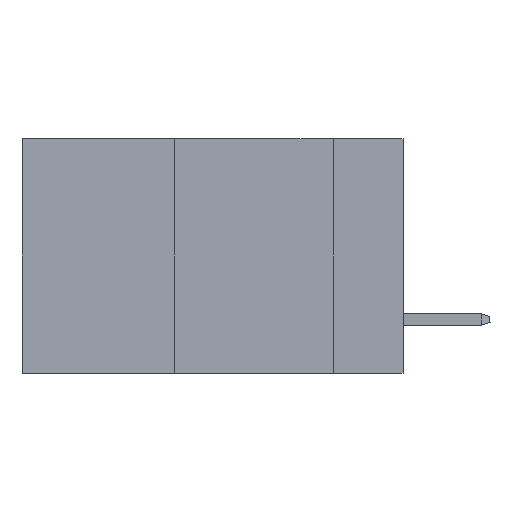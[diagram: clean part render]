
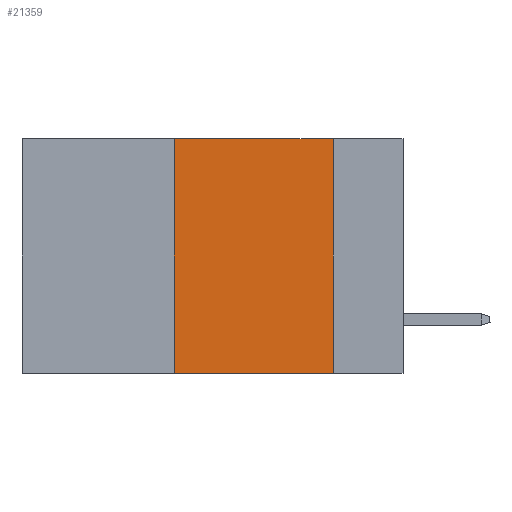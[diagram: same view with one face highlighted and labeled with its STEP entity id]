
A CAD part, left-side view. The second image highlights one B-rep face of the part: STEP entity #21359.
In plain terms, the highlighted planar face has unit normal (-1, 0, 0).
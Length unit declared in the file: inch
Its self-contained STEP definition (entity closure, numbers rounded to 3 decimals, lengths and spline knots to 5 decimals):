
#491 = CARTESIAN_POINT ( 'NONE',  ( 0., 0.36, 0. ) ) ;
#593 = CARTESIAN_POINT ( 'NONE',  ( 0., 0.6, -0.37 ) ) ;
#885 = ORIENTED_EDGE ( 'NONE', *, *, #23435, .F. ) ;
#1419 = CARTESIAN_POINT ( 'NONE',  ( 0., 0.36, 0. ) ) ;
#1528 = LINE ( 'NONE', #17895, #15842 ) ;
#1784 = VERTEX_POINT ( 'NONE', #1419 ) ;
#2158 = EDGE_CURVE ( 'NONE', #2268, #11792, #1528, .T. ) ;
#2268 = VERTEX_POINT ( 'NONE', #6514 ) ;
#4286 = DIRECTION ( 'NONE',  ( 1., 0., 0. ) ) ;
#4711 = LINE ( 'NONE', #491, #28111 ) ;
#5995 = LINE ( 'NONE', #21917, #21559 ) ;
#6258 = FACE_OUTER_BOUND ( 'NONE', #28922, .T. ) ;
#6408 = PLANE ( 'NONE',  #7653 ) ;
#6514 = CARTESIAN_POINT ( 'NONE',  ( 0., 0.11, 0. ) ) ;
#6972 = CARTESIAN_POINT ( 'NONE',  ( 0., 0.36, -0.37 ) ) ;
#7653 = AXIS2_PLACEMENT_3D ( 'NONE', #27317, #4286, #13547 ) ;
#10105 = ORIENTED_EDGE ( 'NONE', *, *, #13487, .T. ) ;
#11792 = VERTEX_POINT ( 'NONE', #20939 ) ;
#13487 = EDGE_CURVE ( 'NONE', #27626, #11792, #21338, .T. ) ;
#13547 = DIRECTION ( 'NONE',  ( 0., 0., -1. ) ) ;
#15261 = DIRECTION ( 'NONE',  ( 0., -1., 0. ) ) ;
#15842 = VECTOR ( 'NONE', #21977, 39.37008 ) ;
#17232 = VECTOR ( 'NONE', #28291, 39.37008 ) ;
#17763 = EDGE_CURVE ( 'NONE', #27626, #1784, #4711, .T. ) ;
#17895 = CARTESIAN_POINT ( 'NONE',  ( 0., 0.11, 0. ) ) ;
#20939 = CARTESIAN_POINT ( 'NONE',  ( 0., 0.11, -0.37 ) ) ;
#21338 = LINE ( 'NONE', #593, #17232 ) ;
#21359 = ADVANCED_FACE ( 'NONE', ( #6258 ), #6408, .F. ) ;
#21559 = VECTOR ( 'NONE', #15261, 39.37008 ) ;
#21917 = CARTESIAN_POINT ( 'NONE',  ( 0., 0.6, 0. ) ) ;
#21977 = DIRECTION ( 'NONE',  ( 0., 0., -1. ) ) ;
#22961 = ORIENTED_EDGE ( 'NONE', *, *, #2158, .F. ) ;
#23435 = EDGE_CURVE ( 'NONE', #1784, #2268, #5995, .T. ) ;
#26174 = ORIENTED_EDGE ( 'NONE', *, *, #17763, .F. ) ;
#27317 = CARTESIAN_POINT ( 'NONE',  ( 0., 0.6, 0. ) ) ;
#27626 = VERTEX_POINT ( 'NONE', #6972 ) ;
#27900 = DIRECTION ( 'NONE',  ( 0., 0., 1. ) ) ;
#28111 = VECTOR ( 'NONE', #27900, 39.37008 ) ;
#28291 = DIRECTION ( 'NONE',  ( 0., -1., 0. ) ) ;
#28922 = EDGE_LOOP ( 'NONE', ( #22961, #885, #26174, #10105 ) ) ;
